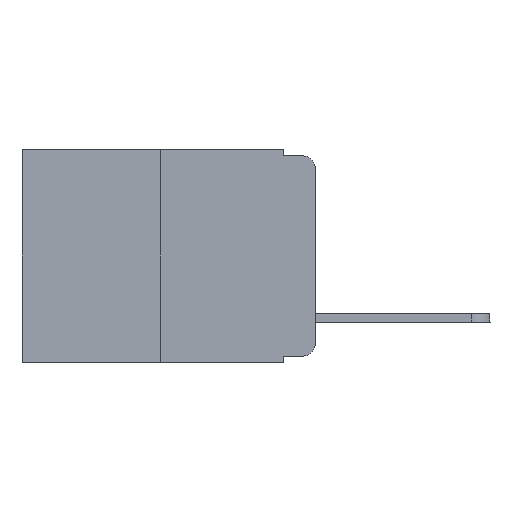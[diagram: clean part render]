
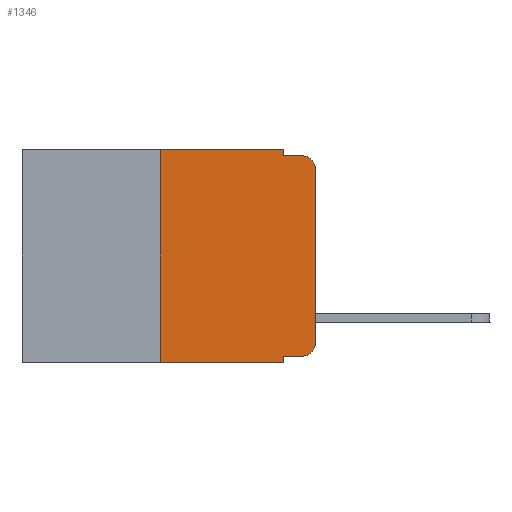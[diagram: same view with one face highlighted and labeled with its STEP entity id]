
A CAD part, left-side view. The second image highlights one B-rep face of the part: STEP entity #1346.
In plain terms, the highlighted planar face has unit normal (-1, 0, 0).
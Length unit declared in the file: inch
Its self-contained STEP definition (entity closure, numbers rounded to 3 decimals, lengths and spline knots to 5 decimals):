
#34 = CARTESIAN_POINT ( 'NONE',  ( 0., 0.25, 0. ) ) ;
#64 = VECTOR ( 'NONE', #3845, 39.37008 ) ;
#342 = EDGE_LOOP ( 'NONE', ( #8453, #8115, #9380, #7625, #5373, #11129, #1487, #1098, #5573, #2247 ) ) ;
#418 = DIRECTION ( 'NONE',  ( 0., 0., 1. ) ) ;
#422 = DIRECTION ( 'NONE',  ( 0., -1., 0. ) ) ;
#425 = CARTESIAN_POINT ( 'NONE',  ( 0., 0.02, -0.313 ) ) ;
#537 = EDGE_CURVE ( 'NONE', #1143, #7083, #5374, .T. ) ;
#696 = EDGE_CURVE ( 'NONE', #6338, #7732, #10653, .T. ) ;
#1050 = AXIS2_PLACEMENT_3D ( 'NONE', #7222, #6425, #3684 ) ;
#1069 = AXIS2_PLACEMENT_3D ( 'NONE', #11601, #5998, #6936 ) ;
#1098 = ORIENTED_EDGE ( 'NONE', *, *, #11004, .F. ) ;
#1143 = VERTEX_POINT ( 'NONE', #3804 ) ;
#1224 = VERTEX_POINT ( 'NONE', #3893 ) ;
#1346 = ADVANCED_FACE ( 'NONE', ( #3426 ), #3439, .F. ) ;
#1487 = ORIENTED_EDGE ( 'NONE', *, *, #10875, .T. ) ;
#1769 = CIRCLE ( 'NONE', #6514, 0.02 ) ;
#2247 = ORIENTED_EDGE ( 'NONE', *, *, #4395, .T. ) ;
#2287 = CARTESIAN_POINT ( 'NONE',  ( 0., 0.051, -0.01 ) ) ;
#2391 = CARTESIAN_POINT ( 'NONE',  ( 0., 0.473, 0. ) ) ;
#2675 = VECTOR ( 'NONE', #5305, 39.37008 ) ;
#3172 = CARTESIAN_POINT ( 'NONE',  ( 0., 0., 0. ) ) ;
#3216 = CARTESIAN_POINT ( 'NONE',  ( 0., 0.051, -0.343 ) ) ;
#3426 = FACE_OUTER_BOUND ( 'NONE', #342, .T. ) ;
#3439 = PLANE ( 'NONE',  #1050 ) ;
#3684 = DIRECTION ( 'NONE',  ( 0., 0., -1. ) ) ;
#3804 = CARTESIAN_POINT ( 'NONE',  ( 0., 0.051, 0. ) ) ;
#3845 = DIRECTION ( 'NONE',  ( 0., 0., -1. ) ) ;
#3893 = CARTESIAN_POINT ( 'NONE',  ( 0., 0.051, -0.333 ) ) ;
#4107 = VECTOR ( 'NONE', #422, 39.37008 ) ;
#4291 = EDGE_CURVE ( 'NONE', #7732, #8371, #8546, .T. ) ;
#4347 = CARTESIAN_POINT ( 'NONE',  ( 0., 0.25, 0. ) ) ;
#4395 = EDGE_CURVE ( 'NONE', #7563, #6338, #1769, .T. ) ;
#4628 = VECTOR ( 'NONE', #418, 39.37008 ) ;
#4806 = EDGE_CURVE ( 'NONE', #7535, #1143, #11170, .T. ) ;
#4869 = CARTESIAN_POINT ( 'NONE',  ( 0., 0.02, -0.01 ) ) ;
#4988 = VECTOR ( 'NONE', #11793, 39.37008 ) ;
#4992 = CARTESIAN_POINT ( 'NONE',  ( 0., 0., -0.313 ) ) ;
#5305 = DIRECTION ( 'NONE',  ( 0., 0., 1. ) ) ;
#5334 = LINE ( 'NONE', #4347, #2675 ) ;
#5373 = ORIENTED_EDGE ( 'NONE', *, *, #4806, .F. ) ;
#5374 = LINE ( 'NONE', #11444, #64 ) ;
#5573 = ORIENTED_EDGE ( 'NONE', *, *, #7310, .T. ) ;
#5647 = CARTESIAN_POINT ( 'NONE',  ( 0., 0.02, -0.333 ) ) ;
#5959 = CARTESIAN_POINT ( 'NONE',  ( 0., 0., -0.03 ) ) ;
#5998 = DIRECTION ( 'NONE',  ( -1., 0., 0. ) ) ;
#6338 = VERTEX_POINT ( 'NONE', #4992 ) ;
#6425 = DIRECTION ( 'NONE',  ( 1., 0., 0. ) ) ;
#6514 = AXIS2_PLACEMENT_3D ( 'NONE', #425, #10814, #9754 ) ;
#6936 = DIRECTION ( 'NONE',  ( 0., 0., -1. ) ) ;
#7083 = VERTEX_POINT ( 'NONE', #2287 ) ;
#7222 = CARTESIAN_POINT ( 'NONE',  ( 0., 0.473, 0. ) ) ;
#7278 = DIRECTION ( 'NONE',  ( 0., -1., 0. ) ) ;
#7310 = EDGE_CURVE ( 'NONE', #1224, #7563, #9707, .T. ) ;
#7375 = LINE ( 'NONE', #7707, #11028 ) ;
#7535 = VERTEX_POINT ( 'NONE', #34 ) ;
#7563 = VERTEX_POINT ( 'NONE', #5647 ) ;
#7625 = ORIENTED_EDGE ( 'NONE', *, *, #537, .F. ) ;
#7707 = CARTESIAN_POINT ( 'NONE',  ( 0., 0.051, -0.01 ) ) ;
#7732 = VERTEX_POINT ( 'NONE', #5959 ) ;
#8067 = VERTEX_POINT ( 'NONE', #9154 ) ;
#8115 = ORIENTED_EDGE ( 'NONE', *, *, #4291, .T. ) ;
#8371 = VERTEX_POINT ( 'NONE', #4869 ) ;
#8453 = ORIENTED_EDGE ( 'NONE', *, *, #696, .T. ) ;
#8536 = LINE ( 'NONE', #9792, #4107 ) ;
#8546 = CIRCLE ( 'NONE', #1069, 0.02 ) ;
#8994 = VECTOR ( 'NONE', #7278, 39.37008 ) ;
#9083 = VERTEX_POINT ( 'NONE', #3216 ) ;
#9154 = CARTESIAN_POINT ( 'NONE',  ( 0., 0.25, -0.343 ) ) ;
#9175 = CARTESIAN_POINT ( 'NONE',  ( 0., 0.051, -0.333 ) ) ;
#9266 = LINE ( 'NONE', #9914, #4988 ) ;
#9380 = ORIENTED_EDGE ( 'NONE', *, *, #10610, .F. ) ;
#9400 = DIRECTION ( 'NONE',  ( 0., -1., 0. ) ) ;
#9687 = VECTOR ( 'NONE', #11707, 39.37008 ) ;
#9707 = LINE ( 'NONE', #9175, #8994 ) ;
#9754 = DIRECTION ( 'NONE',  ( 0., 0., -1. ) ) ;
#9792 = CARTESIAN_POINT ( 'NONE',  ( 0., 0.473, -0.343 ) ) ;
#9833 = EDGE_CURVE ( 'NONE', #8067, #7535, #5334, .T. ) ;
#9914 = CARTESIAN_POINT ( 'NONE',  ( 0., 0.051, 0. ) ) ;
#10610 = EDGE_CURVE ( 'NONE', #7083, #8371, #7375, .T. ) ;
#10653 = LINE ( 'NONE', #3172, #4628 ) ;
#10814 = DIRECTION ( 'NONE',  ( -1., 0., 0. ) ) ;
#10875 = EDGE_CURVE ( 'NONE', #8067, #9083, #8536, .T. ) ;
#11004 = EDGE_CURVE ( 'NONE', #1224, #9083, #9266, .T. ) ;
#11028 = VECTOR ( 'NONE', #9400, 39.37008 ) ;
#11129 = ORIENTED_EDGE ( 'NONE', *, *, #9833, .F. ) ;
#11170 = LINE ( 'NONE', #2391, #9687 ) ;
#11444 = CARTESIAN_POINT ( 'NONE',  ( 0., 0.051, 0. ) ) ;
#11601 = CARTESIAN_POINT ( 'NONE',  ( 0., 0.02, -0.03 ) ) ;
#11707 = DIRECTION ( 'NONE',  ( 0., -1., 0. ) ) ;
#11793 = DIRECTION ( 'NONE',  ( 0., 0., -1. ) ) ;
